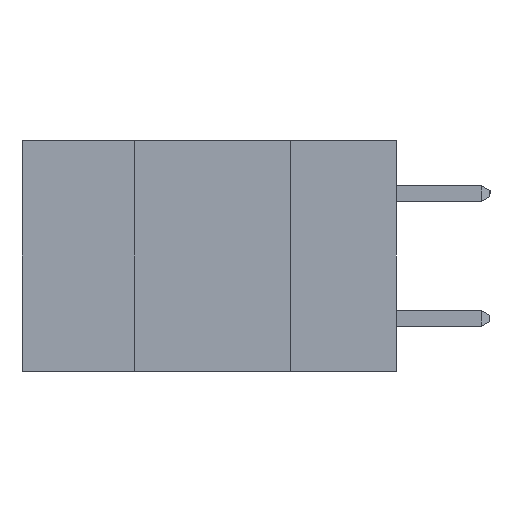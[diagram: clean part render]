
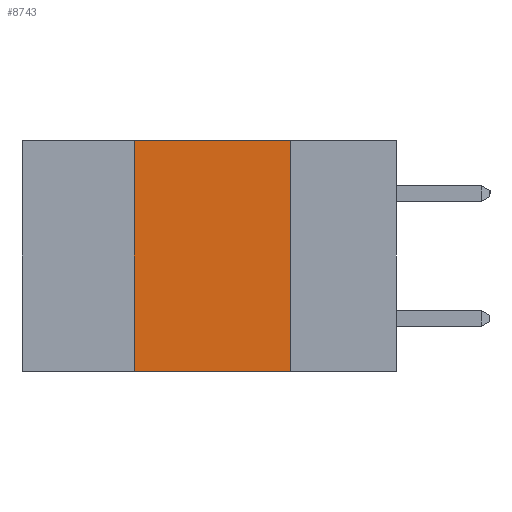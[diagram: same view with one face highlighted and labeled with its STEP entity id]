
A CAD part, left-side view. The second image highlights one B-rep face of the part: STEP entity #8743.
In plain terms, the highlighted planar face has unit normal (-1, 0, 0).
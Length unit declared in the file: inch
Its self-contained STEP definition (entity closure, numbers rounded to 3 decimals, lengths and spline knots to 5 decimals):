
#279 = VECTOR ( 'NONE', #5960, 39.37008 ) ;
#739 = VERTEX_POINT ( 'NONE', #5959 ) ;
#748 = VERTEX_POINT ( 'NONE', #3521 ) ;
#1246 = LINE ( 'NONE', #9634, #1312 ) ;
#1312 = VECTOR ( 'NONE', #7938, 39.37008 ) ;
#1546 = DIRECTION ( 'NONE',  ( 0., 0., -1. ) ) ;
#1815 = EDGE_CURVE ( 'NONE', #4920, #748, #7727, .T. ) ;
#2201 = CARTESIAN_POINT ( 'NONE',  ( 0., 0.6, 0. ) ) ;
#2691 = CARTESIAN_POINT ( 'NONE',  ( 0., 0.42, -0.37 ) ) ;
#2824 = ORIENTED_EDGE ( 'NONE', *, *, #9046, .F. ) ;
#2973 = DIRECTION ( 'NONE',  ( 1., 0., 0. ) ) ;
#3463 = CARTESIAN_POINT ( 'NONE',  ( 0., 0.17, 0. ) ) ;
#3521 = CARTESIAN_POINT ( 'NONE',  ( 0., 0.17, -0.37 ) ) ;
#3743 = PLANE ( 'NONE',  #9265 ) ;
#3800 = VERTEX_POINT ( 'NONE', #3463 ) ;
#4606 = ORIENTED_EDGE ( 'NONE', *, *, #8646, .F. ) ;
#4694 = FACE_OUTER_BOUND ( 'NONE', #10885, .T. ) ;
#4863 = LINE ( 'NONE', #9974, #5051 ) ;
#4920 = VERTEX_POINT ( 'NONE', #5747 ) ;
#5051 = VECTOR ( 'NONE', #1546, 39.37008 ) ;
#5747 = CARTESIAN_POINT ( 'NONE',  ( 0., 0.42, -0.37 ) ) ;
#5959 = CARTESIAN_POINT ( 'NONE',  ( 0., 0.42, 0. ) ) ;
#5960 = DIRECTION ( 'NONE',  ( 0., 0., 1. ) ) ;
#6064 = DIRECTION ( 'NONE',  ( 0., -1., 0. ) ) ;
#6234 = DIRECTION ( 'NONE',  ( 0., 0., -1. ) ) ;
#6480 = VECTOR ( 'NONE', #6064, 39.37008 ) ;
#7076 = ORIENTED_EDGE ( 'NONE', *, *, #8863, .F. ) ;
#7727 = LINE ( 'NONE', #8657, #6480 ) ;
#7938 = DIRECTION ( 'NONE',  ( 0., -1., 0. ) ) ;
#8646 = EDGE_CURVE ( 'NONE', #739, #3800, #1246, .T. ) ;
#8657 = CARTESIAN_POINT ( 'NONE',  ( 0., 0.6, -0.37 ) ) ;
#8743 = ADVANCED_FACE ( 'NONE', ( #4694 ), #3743, .F. ) ;
#8863 = EDGE_CURVE ( 'NONE', #3800, #748, #4863, .T. ) ;
#9046 = EDGE_CURVE ( 'NONE', #4920, #739, #9266, .T. ) ;
#9265 = AXIS2_PLACEMENT_3D ( 'NONE', #2201, #2973, #6234 ) ;
#9266 = LINE ( 'NONE', #2691, #279 ) ;
#9436 = ORIENTED_EDGE ( 'NONE', *, *, #1815, .T. ) ;
#9634 = CARTESIAN_POINT ( 'NONE',  ( 0., 0.6, 0. ) ) ;
#9974 = CARTESIAN_POINT ( 'NONE',  ( 0., 0.17, -0.37 ) ) ;
#10885 = EDGE_LOOP ( 'NONE', ( #7076, #4606, #2824, #9436 ) ) ;
